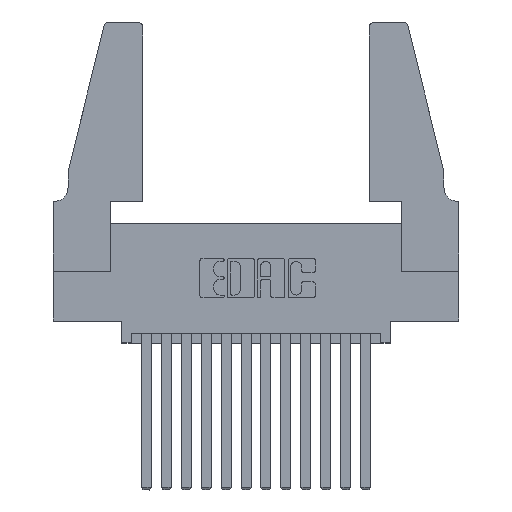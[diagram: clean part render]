
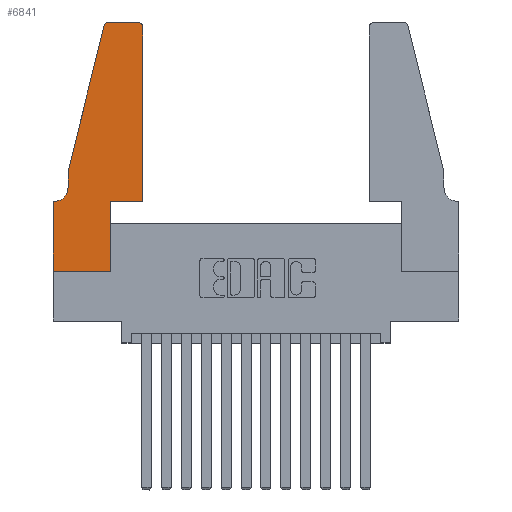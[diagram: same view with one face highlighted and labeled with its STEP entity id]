
A CAD part, top view. The second image highlights one B-rep face of the part: STEP entity #6841.
In plain terms, the highlighted planar face has unit normal (0, 0, 1).
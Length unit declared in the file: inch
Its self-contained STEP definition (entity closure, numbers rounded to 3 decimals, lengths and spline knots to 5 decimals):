
#155 = EDGE_LOOP ( 'NONE', ( #14131, #4932, #13694, #8356, #364, #6992, #14684, #2011, #7334, #11689, #6695, #660 ) ) ;
#216 = CARTESIAN_POINT ( 'NONE',  ( 0., 0., 0.37 ) ) ;
#279 = DIRECTION ( 'NONE',  ( 0., 0., 1. ) ) ;
#288 = CARTESIAN_POINT ( 'NONE',  ( 0.2605, 1.25, 0.37 ) ) ;
#364 = ORIENTED_EDGE ( 'NONE', *, *, #6912, .T. ) ;
#377 = VERTEX_POINT ( 'NONE', #10619 ) ;
#616 = VERTEX_POINT ( 'NONE', #11906 ) ;
#660 = ORIENTED_EDGE ( 'NONE', *, *, #13234, .T. ) ;
#1027 = DIRECTION ( 'NONE',  ( 0., 0., 1. ) ) ;
#1084 = EDGE_CURVE ( 'NONE', #12099, #377, #11097, .T. ) ;
#1104 = EDGE_CURVE ( 'NONE', #5166, #12099, #10156, .T. ) ;
#1122 = DIRECTION ( 'NONE',  ( 0., 0., 1. ) ) ;
#1227 = VECTOR ( 'NONE', #2180, 39.37008 ) ;
#1413 = LINE ( 'NONE', #5828, #10575 ) ;
#1510 = AXIS2_PLACEMENT_3D ( 'NONE', #9399, #1027, #4926 ) ;
#1816 = AXIS2_PLACEMENT_3D ( 'NONE', #5426, #10166, #7876 ) ;
#1828 = VERTEX_POINT ( 'NONE', #10561 ) ;
#2011 = ORIENTED_EDGE ( 'NONE', *, *, #11252, .T. ) ;
#2143 = DIRECTION ( 'NONE',  ( -0.239, -0.971, 0. ) ) ;
#2180 = DIRECTION ( 'NONE',  ( 0., 1., 0. ) ) ;
#2594 = CARTESIAN_POINT ( 'NONE',  ( 0.284, 1.25, 0.37 ) ) ;
#3088 = DIRECTION ( 'NONE',  ( 0., -1., 0. ) ) ;
#3140 = CIRCLE ( 'NONE', #8389, 0.03 ) ;
#3455 = CARTESIAN_POINT ( 'NONE',  ( 0.4205, 1.22, 0.37 ) ) ;
#3756 = LINE ( 'NONE', #216, #9029 ) ;
#3765 = LINE ( 'NONE', #4500, #14528 ) ;
#3887 = VERTEX_POINT ( 'NONE', #9457 ) ;
#4289 = VECTOR ( 'NONE', #3088, 39.37008 ) ;
#4500 = CARTESIAN_POINT ( 'NONE',  ( 0.4505, 0.35, 0.37 ) ) ;
#4651 = DIRECTION ( 'NONE',  ( 1., 0., 0. ) ) ;
#4858 = DIRECTION ( 'NONE',  ( 1., 0., 0. ) ) ;
#4926 = DIRECTION ( 'NONE',  ( 1., 0., 0. ) ) ;
#4932 = ORIENTED_EDGE ( 'NONE', *, *, #1104, .T. ) ;
#5166 = VERTEX_POINT ( 'NONE', #2594 ) ;
#5209 = EDGE_CURVE ( 'NONE', #616, #5166, #9465, .T. ) ;
#5426 = CARTESIAN_POINT ( 'NONE',  ( 0.0055, 0.42, 0.37 ) ) ;
#5474 = CIRCLE ( 'NONE', #1816, 0.07 ) ;
#5775 = DIRECTION ( 'NONE',  ( 0., -1., 0. ) ) ;
#5828 = CARTESIAN_POINT ( 'NONE',  ( 0.0755, 0.5, 0.37 ) ) ;
#5977 = CARTESIAN_POINT ( 'NONE',  ( 0.0755, 0.42, 0.37 ) ) ;
#6274 = CARTESIAN_POINT ( 'NONE',  ( 0.2865, 0.35, 0.37 ) ) ;
#6295 = VERTEX_POINT ( 'NONE', #10240 ) ;
#6527 = CARTESIAN_POINT ( 'NONE',  ( 0., 0., 0.37 ) ) ;
#6581 = EDGE_CURVE ( 'NONE', #9287, #6295, #3765, .T. ) ;
#6695 = ORIENTED_EDGE ( 'NONE', *, *, #14043, .T. ) ;
#6722 = DIRECTION ( 'NONE',  ( -1., 0., 0. ) ) ;
#6792 = VERTEX_POINT ( 'NONE', #9744 ) ;
#6841 = ADVANCED_FACE ( 'NONE', ( #14333 ), #14678, .T. ) ;
#6912 = EDGE_CURVE ( 'NONE', #10906, #8888, #5474, .T. ) ;
#6992 = ORIENTED_EDGE ( 'NONE', *, *, #7010, .T. ) ;
#7010 = EDGE_CURVE ( 'NONE', #8888, #1828, #10924, .T. ) ;
#7334 = ORIENTED_EDGE ( 'NONE', *, *, #14876, .T. ) ;
#7487 = CARTESIAN_POINT ( 'NONE',  ( 0., 0.35, 0.37 ) ) ;
#7775 = VECTOR ( 'NONE', #6722, 39.37008 ) ;
#7876 = DIRECTION ( 'NONE',  ( -1., 0., 0. ) ) ;
#8356 = ORIENTED_EDGE ( 'NONE', *, *, #15301, .T. ) ;
#8389 = AXIS2_PLACEMENT_3D ( 'NONE', #3455, #1122, #4651 ) ;
#8479 = VECTOR ( 'NONE', #2143, 39.37008 ) ;
#8601 = CARTESIAN_POINT ( 'NONE',  ( 0.0055, 0.35, 0.37 ) ) ;
#8608 = DIRECTION ( 'NONE',  ( -1., 0., 0. ) ) ;
#8888 = VERTEX_POINT ( 'NONE', #8601 ) ;
#9029 = VECTOR ( 'NONE', #9031, 39.37008 ) ;
#9031 = DIRECTION ( 'NONE',  ( 1., 0., 0. ) ) ;
#9287 = VERTEX_POINT ( 'NONE', #6274 ) ;
#9296 = CARTESIAN_POINT ( 'NONE',  ( 0.0755, 0.5, 0.37 ) ) ;
#9364 = CARTESIAN_POINT ( 'NONE',  ( 0.4505, 0.35, 0.37 ) ) ;
#9399 = CARTESIAN_POINT ( 'NONE',  ( 0.284, 1.22, 0.37 ) ) ;
#9457 = CARTESIAN_POINT ( 'NONE',  ( 0.4505, 1.22, 0.37 ) ) ;
#9465 = LINE ( 'NONE', #288, #12851 ) ;
#9744 = CARTESIAN_POINT ( 'NONE',  ( 0., 0., 0.37 ) ) ;
#10156 = CIRCLE ( 'NONE', #1510, 0.03 ) ;
#10166 = DIRECTION ( 'NONE',  ( 0., 0., -1. ) ) ;
#10240 = CARTESIAN_POINT ( 'NONE',  ( 0.4505, 0.35, 0.37 ) ) ;
#10434 = VECTOR ( 'NONE', #15403, 39.37008 ) ;
#10561 = CARTESIAN_POINT ( 'NONE',  ( 0., 0.35, 0.37 ) ) ;
#10575 = VECTOR ( 'NONE', #5775, 39.37008 ) ;
#10619 = CARTESIAN_POINT ( 'NONE',  ( 0.0755, 0.5, 0.37 ) ) ;
#10906 = VERTEX_POINT ( 'NONE', #5977 ) ;
#10924 = LINE ( 'NONE', #11110, #7775 ) ;
#11097 = LINE ( 'NONE', #9296, #8479 ) ;
#11110 = CARTESIAN_POINT ( 'NONE',  ( 0.0755, 0.35, 0.37 ) ) ;
#11252 = EDGE_CURVE ( 'NONE', #6792, #14453, #3756, .T. ) ;
#11689 = ORIENTED_EDGE ( 'NONE', *, *, #6581, .T. ) ;
#11815 = EDGE_CURVE ( 'NONE', #1828, #6792, #14280, .T. ) ;
#11906 = CARTESIAN_POINT ( 'NONE',  ( 0.4205, 1.25, 0.37 ) ) ;
#12099 = VERTEX_POINT ( 'NONE', #15081 ) ;
#12668 = CARTESIAN_POINT ( 'NONE',  ( 0.2865, 0., 0.37 ) ) ;
#12851 = VECTOR ( 'NONE', #8608, 39.37008 ) ;
#13234 = EDGE_CURVE ( 'NONE', #3887, #616, #3140, .T. ) ;
#13658 = LINE ( 'NONE', #9364, #10434 ) ;
#13694 = ORIENTED_EDGE ( 'NONE', *, *, #1084, .T. ) ;
#14043 = EDGE_CURVE ( 'NONE', #6295, #3887, #13658, .T. ) ;
#14131 = ORIENTED_EDGE ( 'NONE', *, *, #5209, .T. ) ;
#14149 = LINE ( 'NONE', #14653, #1227 ) ;
#14170 = AXIS2_PLACEMENT_3D ( 'NONE', #7487, #279, #4858 ) ;
#14280 = LINE ( 'NONE', #6527, #4289 ) ;
#14333 = FACE_OUTER_BOUND ( 'NONE', #155, .T. ) ;
#14453 = VERTEX_POINT ( 'NONE', #12668 ) ;
#14528 = VECTOR ( 'NONE', #15175, 39.37008 ) ;
#14653 = CARTESIAN_POINT ( 'NONE',  ( 0.2865, 0.35, 0.37 ) ) ;
#14678 = PLANE ( 'NONE',  #14170 ) ;
#14684 = ORIENTED_EDGE ( 'NONE', *, *, #11815, .T. ) ;
#14876 = EDGE_CURVE ( 'NONE', #14453, #9287, #14149, .T. ) ;
#15081 = CARTESIAN_POINT ( 'NONE',  ( 0.25487, 1.22718, 0.37 ) ) ;
#15175 = DIRECTION ( 'NONE',  ( 1., 0., 0. ) ) ;
#15301 = EDGE_CURVE ( 'NONE', #377, #10906, #1413, .T. ) ;
#15403 = DIRECTION ( 'NONE',  ( 0., 1., 0. ) ) ;
